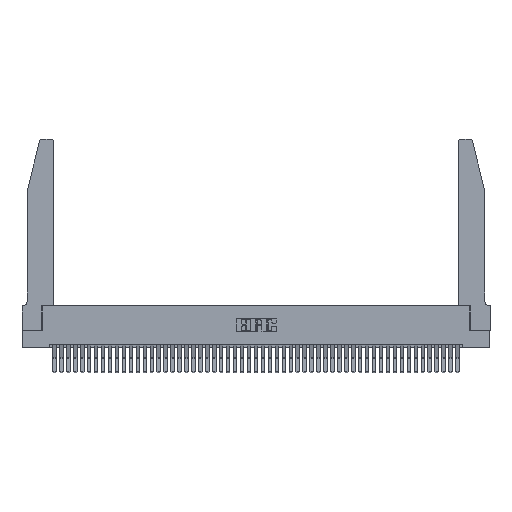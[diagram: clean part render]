
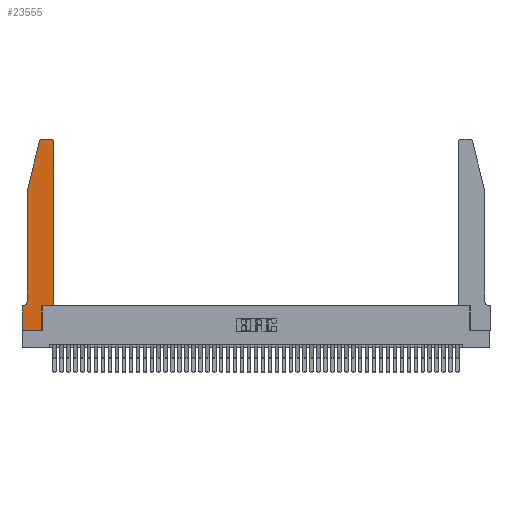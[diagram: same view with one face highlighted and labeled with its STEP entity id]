
A CAD part, top view. The second image highlights one B-rep face of the part: STEP entity #23555.
In plain terms, the highlighted planar face has unit normal (0, 0, 1).
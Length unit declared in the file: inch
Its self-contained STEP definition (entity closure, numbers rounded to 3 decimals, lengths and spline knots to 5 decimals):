
#638 = ORIENTED_EDGE ( 'NONE', *, *, #10450, .T. ) ;
#1140 = CIRCLE ( 'NONE', #20329, 0.03 ) ;
#1449 = ORIENTED_EDGE ( 'NONE', *, *, #2318, .T. ) ;
#2318 = EDGE_CURVE ( 'NONE', #43433, #10350, #46971, .T. ) ;
#2850 = AXIS2_PLACEMENT_3D ( 'NONE', #10130, #36337, #43624 ) ;
#3766 = LINE ( 'NONE', #13715, #14386 ) ;
#4645 = ORIENTED_EDGE ( 'NONE', *, *, #37385, .T. ) ;
#6418 = LINE ( 'NONE', #27130, #31750 ) ;
#7412 = VECTOR ( 'NONE', #37910, 39.37008 ) ;
#7612 = CARTESIAN_POINT ( 'NONE',  ( 0.0755, 0.42, 0.37 ) ) ;
#8213 = DIRECTION ( 'NONE',  ( 0., -1., 0. ) ) ;
#8430 = VERTEX_POINT ( 'NONE', #16213 ) ;
#8777 = EDGE_CURVE ( 'NONE', #33555, #8430, #3766, .T. ) ;
#9159 = DIRECTION ( 'NONE',  ( 1., 0., 0. ) ) ;
#9180 = CARTESIAN_POINT ( 'NONE',  ( 0.2865, 0., 0.37 ) ) ;
#9551 = LINE ( 'NONE', #13411, #29612 ) ;
#10072 = CARTESIAN_POINT ( 'NONE',  ( 0.4505, 0.35, 0.37 ) ) ;
#10130 = CARTESIAN_POINT ( 'NONE',  ( 0.4205, 2.72, 0.37 ) ) ;
#10350 = VERTEX_POINT ( 'NONE', #24073 ) ;
#10450 = EDGE_CURVE ( 'NONE', #36579, #37967, #6418, .T. ) ;
#11243 = CARTESIAN_POINT ( 'NONE',  ( 0.0055, 0.42, 0.37 ) ) ;
#11331 = ORIENTED_EDGE ( 'NONE', *, *, #40688, .T. ) ;
#12645 = PLANE ( 'NONE',  #45607 ) ;
#13411 = CARTESIAN_POINT ( 'NONE',  ( 0.2865, 0.35, 0.37 ) ) ;
#13715 = CARTESIAN_POINT ( 'NONE',  ( 0.4505, 0.35, 0.37 ) ) ;
#13877 = ORIENTED_EDGE ( 'NONE', *, *, #19003, .T. ) ;
#14386 = VECTOR ( 'NONE', #25579, 39.37008 ) ;
#14685 = DIRECTION ( 'NONE',  ( 0., 0., -1. ) ) ;
#14787 = CARTESIAN_POINT ( 'NONE',  ( 0.0755, 2., 0.37 ) ) ;
#15173 = CARTESIAN_POINT ( 'NONE',  ( 0.0755, 0.35, 0.37 ) ) ;
#15366 = CARTESIAN_POINT ( 'NONE',  ( 0.0755, 2., 0.37 ) ) ;
#16060 = VERTEX_POINT ( 'NONE', #44987 ) ;
#16213 = CARTESIAN_POINT ( 'NONE',  ( 0.4505, 2.72, 0.37 ) ) ;
#17702 = AXIS2_PLACEMENT_3D ( 'NONE', #11243, #14685, #45389 ) ;
#18269 = EDGE_CURVE ( 'NONE', #10350, #48726, #32730, .T. ) ;
#19003 = EDGE_CURVE ( 'NONE', #40173, #33555, #30883, .T. ) ;
#19190 = DIRECTION ( 'NONE',  ( -0.239, -0.971, 0. ) ) ;
#19475 = VERTEX_POINT ( 'NONE', #9180 ) ;
#20018 = ORIENTED_EDGE ( 'NONE', *, *, #31776, .T. ) ;
#20225 = EDGE_CURVE ( 'NONE', #37967, #43433, #45635, .T. ) ;
#20329 = AXIS2_PLACEMENT_3D ( 'NONE', #26247, #29719, #34154 ) ;
#20549 = ORIENTED_EDGE ( 'NONE', *, *, #18269, .T. ) ;
#21879 = EDGE_CURVE ( 'NONE', #19475, #40173, #9551, .T. ) ;
#22749 = VECTOR ( 'NONE', #36614, 39.37008 ) ;
#22799 = CARTESIAN_POINT ( 'NONE',  ( 0.0055, 0.35, 0.37 ) ) ;
#23141 = LINE ( 'NONE', #30485, #31946 ) ;
#23555 = ADVANCED_FACE ( 'NONE', ( #37703 ), #12645, .T. ) ;
#24073 = CARTESIAN_POINT ( 'NONE',  ( 0., 0.35, 0.37 ) ) ;
#24949 = LINE ( 'NONE', #15366, #34403 ) ;
#25579 = DIRECTION ( 'NONE',  ( 0., 1., 0. ) ) ;
#25583 = CARTESIAN_POINT ( 'NONE',  ( 0., 0., 0.37 ) ) ;
#26247 = CARTESIAN_POINT ( 'NONE',  ( 0.284, 2.72, 0.37 ) ) ;
#26911 = EDGE_LOOP ( 'NONE', ( #20018, #11331, #4645, #638, #43659, #1449, #20549, #45457, #39333, #13877, #36599, #29462 ) ) ;
#27130 = CARTESIAN_POINT ( 'NONE',  ( 0.0755, 2., 0.37 ) ) ;
#27786 = CARTESIAN_POINT ( 'NONE',  ( 0., 0.35, 0.37 ) ) ;
#28575 = DIRECTION ( 'NONE',  ( -1., 0., 0. ) ) ;
#29462 = ORIENTED_EDGE ( 'NONE', *, *, #36941, .T. ) ;
#29612 = VECTOR ( 'NONE', #32344, 39.37008 ) ;
#29719 = DIRECTION ( 'NONE',  ( 0., 0., 1. ) ) ;
#30075 = VERTEX_POINT ( 'NONE', #44906 ) ;
#30485 = CARTESIAN_POINT ( 'NONE',  ( 0., 0., 0.37 ) ) ;
#30883 = LINE ( 'NONE', #48302, #33838 ) ;
#31519 = CIRCLE ( 'NONE', #2850, 0.03 ) ;
#31750 = VECTOR ( 'NONE', #8213, 39.37008 ) ;
#31776 = EDGE_CURVE ( 'NONE', #30075, #47432, #46203, .T. ) ;
#31946 = VECTOR ( 'NONE', #34757, 39.37008 ) ;
#32057 = EDGE_CURVE ( 'NONE', #48726, #19475, #23141, .T. ) ;
#32344 = DIRECTION ( 'NONE',  ( 0., 1., 0. ) ) ;
#32730 = LINE ( 'NONE', #25583, #22749 ) ;
#33555 = VERTEX_POINT ( 'NONE', #10072 ) ;
#33838 = VECTOR ( 'NONE', #48144, 39.37008 ) ;
#34154 = DIRECTION ( 'NONE',  ( 1., 0., 0. ) ) ;
#34403 = VECTOR ( 'NONE', #19190, 39.37008 ) ;
#34757 = DIRECTION ( 'NONE',  ( 1., 0., 0. ) ) ;
#36337 = DIRECTION ( 'NONE',  ( 0., 0., 1. ) ) ;
#36579 = VERTEX_POINT ( 'NONE', #14787 ) ;
#36599 = ORIENTED_EDGE ( 'NONE', *, *, #8777, .T. ) ;
#36614 = DIRECTION ( 'NONE',  ( 0., -1., 0. ) ) ;
#36941 = EDGE_CURVE ( 'NONE', #8430, #30075, #31519, .T. ) ;
#37385 = EDGE_CURVE ( 'NONE', #16060, #36579, #24949, .T. ) ;
#37703 = FACE_OUTER_BOUND ( 'NONE', #26911, .T. ) ;
#37910 = DIRECTION ( 'NONE',  ( -1., 0., 0. ) ) ;
#37967 = VERTEX_POINT ( 'NONE', #7612 ) ;
#39333 = ORIENTED_EDGE ( 'NONE', *, *, #21879, .T. ) ;
#39665 = CARTESIAN_POINT ( 'NONE',  ( 0., 0., 0.37 ) ) ;
#40173 = VERTEX_POINT ( 'NONE', #45471 ) ;
#40688 = EDGE_CURVE ( 'NONE', #47432, #16060, #1140, .T. ) ;
#42289 = CARTESIAN_POINT ( 'NONE',  ( 0.284, 2.75, 0.37 ) ) ;
#42976 = DIRECTION ( 'NONE',  ( 0., 0., 1. ) ) ;
#43433 = VERTEX_POINT ( 'NONE', #22799 ) ;
#43624 = DIRECTION ( 'NONE',  ( 1., 0., 0. ) ) ;
#43659 = ORIENTED_EDGE ( 'NONE', *, *, #20225, .T. ) ;
#43932 = CARTESIAN_POINT ( 'NONE',  ( 0.2605, 2.75, 0.37 ) ) ;
#44906 = CARTESIAN_POINT ( 'NONE',  ( 0.4205, 2.75, 0.37 ) ) ;
#44987 = CARTESIAN_POINT ( 'NONE',  ( 0.25487, 2.72718, 0.37 ) ) ;
#45012 = VECTOR ( 'NONE', #28575, 39.37008 ) ;
#45389 = DIRECTION ( 'NONE',  ( -1., 0., 0. ) ) ;
#45457 = ORIENTED_EDGE ( 'NONE', *, *, #32057, .T. ) ;
#45471 = CARTESIAN_POINT ( 'NONE',  ( 0.2865, 0.35, 0.37 ) ) ;
#45607 = AXIS2_PLACEMENT_3D ( 'NONE', #27786, #42976, #9159 ) ;
#45635 = CIRCLE ( 'NONE', #17702, 0.07 ) ;
#46203 = LINE ( 'NONE', #43932, #45012 ) ;
#46971 = LINE ( 'NONE', #15173, #7412 ) ;
#47432 = VERTEX_POINT ( 'NONE', #42289 ) ;
#48144 = DIRECTION ( 'NONE',  ( 1., 0., 0. ) ) ;
#48302 = CARTESIAN_POINT ( 'NONE',  ( 0.4505, 0.35, 0.37 ) ) ;
#48726 = VERTEX_POINT ( 'NONE', #39665 ) ;
